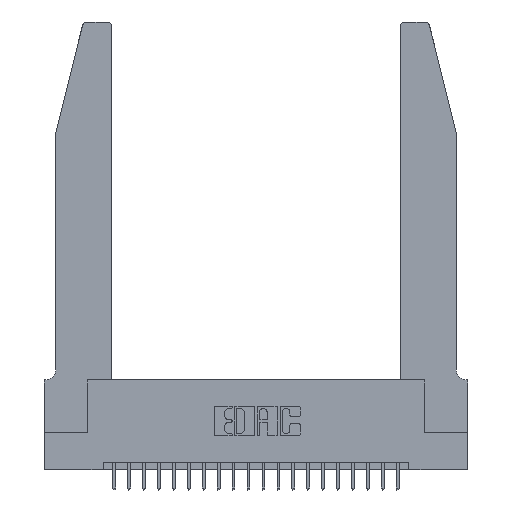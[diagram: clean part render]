
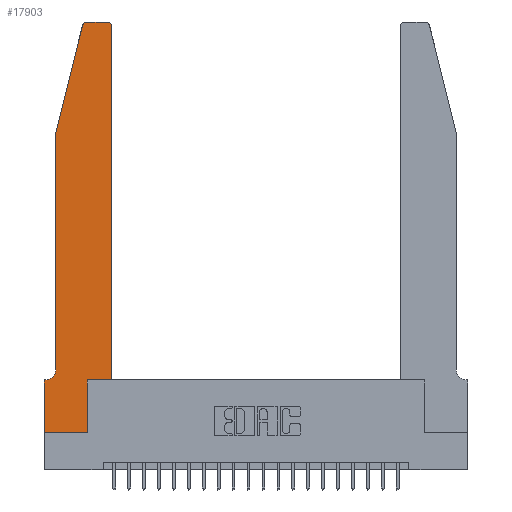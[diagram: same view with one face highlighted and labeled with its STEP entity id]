
A CAD part, top view. The second image highlights one B-rep face of the part: STEP entity #17903.
In plain terms, the highlighted planar face has unit normal (0, 0, 1).
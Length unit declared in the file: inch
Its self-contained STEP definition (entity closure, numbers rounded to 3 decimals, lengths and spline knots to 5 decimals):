
#9 = LINE ( 'NONE', #21988, #9299 ) ;
#37 = CARTESIAN_POINT ( 'NONE',  ( 0.284, 2.75, 0.37 ) ) ;
#168 = AXIS2_PLACEMENT_3D ( 'NONE', #8250, #23098, #8481 ) ;
#295 = AXIS2_PLACEMENT_3D ( 'NONE', #23239, #6489, #6945 ) ;
#527 = CARTESIAN_POINT ( 'NONE',  ( 0.4505, 0.35, 0.37 ) ) ;
#773 = DIRECTION ( 'NONE',  ( 0., -1., 0. ) ) ;
#843 = AXIS2_PLACEMENT_3D ( 'NONE', #21828, #7455, #3656 ) ;
#1049 = VERTEX_POINT ( 'NONE', #18879 ) ;
#1431 = LINE ( 'NONE', #8902, #14630 ) ;
#1601 = EDGE_CURVE ( 'NONE', #4205, #14137, #6245, .T. ) ;
#1781 = EDGE_CURVE ( 'NONE', #13615, #9035, #11203, .T. ) ;
#1956 = DIRECTION ( 'NONE',  ( 1., 0., 0. ) ) ;
#1986 = DIRECTION ( 'NONE',  ( 0., 1., 0. ) ) ;
#2216 = DIRECTION ( 'NONE',  ( 0., 1., 0. ) ) ;
#2668 = LINE ( 'NONE', #19183, #8946 ) ;
#3221 = EDGE_CURVE ( 'NONE', #9035, #3982, #1431, .T. ) ;
#3656 = DIRECTION ( 'NONE',  ( 1., 0., 0. ) ) ;
#3982 = VERTEX_POINT ( 'NONE', #9433 ) ;
#4205 = VERTEX_POINT ( 'NONE', #4580 ) ;
#4580 = CARTESIAN_POINT ( 'NONE',  ( 0.4505, 0.35, 0.37 ) ) ;
#4664 = EDGE_CURVE ( 'NONE', #1049, #4205, #9, .T. ) ;
#4724 = DIRECTION ( 'NONE',  ( 0., -1., 0. ) ) ;
#4725 = VERTEX_POINT ( 'NONE', #9026 ) ;
#5282 = ORIENTED_EDGE ( 'NONE', *, *, #1601, .T. ) ;
#6245 = LINE ( 'NONE', #527, #22203 ) ;
#6339 = VERTEX_POINT ( 'NONE', #8221 ) ;
#6489 = DIRECTION ( 'NONE',  ( 0., 0., 1. ) ) ;
#6945 = DIRECTION ( 'NONE',  ( 1., 0., 0. ) ) ;
#7062 = CARTESIAN_POINT ( 'NONE',  ( 0., 0.35, 0.37 ) ) ;
#7174 = LINE ( 'NONE', #11845, #17744 ) ;
#7227 = EDGE_CURVE ( 'NONE', #6339, #13615, #7174, .T. ) ;
#7356 = DIRECTION ( 'NONE',  ( 1., 0., 0. ) ) ;
#7357 = LINE ( 'NONE', #21075, #20033 ) ;
#7427 = CARTESIAN_POINT ( 'NONE',  ( 0.0755, 0.42, 0.37 ) ) ;
#7455 = DIRECTION ( 'NONE',  ( 0., 0., 1. ) ) ;
#7526 = AXIS2_PLACEMENT_3D ( 'NONE', #7062, #8830, #1956 ) ;
#7940 = EDGE_CURVE ( 'NONE', #14137, #8467, #21160, .T. ) ;
#8045 = CIRCLE ( 'NONE', #843, 0.03 ) ;
#8221 = CARTESIAN_POINT ( 'NONE',  ( 0.0755, 2., 0.37 ) ) ;
#8250 = CARTESIAN_POINT ( 'NONE',  ( 0.0055, 0.42, 0.37 ) ) ;
#8467 = VERTEX_POINT ( 'NONE', #19097 ) ;
#8481 = DIRECTION ( 'NONE',  ( -1., 0., 0. ) ) ;
#8628 = LINE ( 'NONE', #17665, #11826 ) ;
#8756 = ORIENTED_EDGE ( 'NONE', *, *, #1781, .T. ) ;
#8830 = DIRECTION ( 'NONE',  ( 0., 0., 1. ) ) ;
#8902 = CARTESIAN_POINT ( 'NONE',  ( 0.0755, 0.35, 0.37 ) ) ;
#8946 = VECTOR ( 'NONE', #773, 39.37008 ) ;
#9026 = CARTESIAN_POINT ( 'NONE',  ( 0., 0., 0.37 ) ) ;
#9035 = VERTEX_POINT ( 'NONE', #15468 ) ;
#9197 = EDGE_CURVE ( 'NONE', #4725, #21643, #20291, .T. ) ;
#9299 = VECTOR ( 'NONE', #14511, 39.37008 ) ;
#9433 = CARTESIAN_POINT ( 'NONE',  ( 0., 0.35, 0.37 ) ) ;
#9518 = VECTOR ( 'NONE', #20572, 39.37008 ) ;
#10030 = EDGE_LOOP ( 'NONE', ( #13180, #12534, #22954, #17304, #8756, #23449, #12847, #22909, #19371, #20914, #5282, #10141 ) ) ;
#10141 = ORIENTED_EDGE ( 'NONE', *, *, #7940, .T. ) ;
#10971 = VECTOR ( 'NONE', #7356, 39.37008 ) ;
#11203 = CIRCLE ( 'NONE', #168, 0.07 ) ;
#11826 = VECTOR ( 'NONE', #1986, 39.37008 ) ;
#11845 = CARTESIAN_POINT ( 'NONE',  ( 0.0755, 2., 0.37 ) ) ;
#12018 = DIRECTION ( 'NONE',  ( -1., 0., 0. ) ) ;
#12534 = ORIENTED_EDGE ( 'NONE', *, *, #14571, .T. ) ;
#12847 = ORIENTED_EDGE ( 'NONE', *, *, #15275, .T. ) ;
#13180 = ORIENTED_EDGE ( 'NONE', *, *, #23106, .T. ) ;
#13610 = DIRECTION ( 'NONE',  ( -0.239, -0.971, 0. ) ) ;
#13615 = VERTEX_POINT ( 'NONE', #7427 ) ;
#13830 = EDGE_CURVE ( 'NONE', #21643, #1049, #8628, .T. ) ;
#13940 = CARTESIAN_POINT ( 'NONE',  ( 0.2865, 0., 0.37 ) ) ;
#14137 = VERTEX_POINT ( 'NONE', #20413 ) ;
#14424 = FACE_OUTER_BOUND ( 'NONE', #10030, .T. ) ;
#14511 = DIRECTION ( 'NONE',  ( 1., 0., 0. ) ) ;
#14571 = EDGE_CURVE ( 'NONE', #15580, #19890, #8045, .T. ) ;
#14630 = VECTOR ( 'NONE', #12018, 39.37008 ) ;
#15275 = EDGE_CURVE ( 'NONE', #3982, #4725, #2668, .T. ) ;
#15468 = CARTESIAN_POINT ( 'NONE',  ( 0.0055, 0.35, 0.37 ) ) ;
#15580 = VERTEX_POINT ( 'NONE', #37 ) ;
#17008 = LINE ( 'NONE', #22490, #9518 ) ;
#17304 = ORIENTED_EDGE ( 'NONE', *, *, #7227, .T. ) ;
#17665 = CARTESIAN_POINT ( 'NONE',  ( 0.2865, 0.35, 0.37 ) ) ;
#17728 = EDGE_CURVE ( 'NONE', #19890, #6339, #7357, .T. ) ;
#17744 = VECTOR ( 'NONE', #4724, 39.37008 ) ;
#17903 = ADVANCED_FACE ( 'NONE', ( #14424 ), #18104, .T. ) ;
#18104 = PLANE ( 'NONE',  #7526 ) ;
#18160 = CARTESIAN_POINT ( 'NONE',  ( 0., 0., 0.37 ) ) ;
#18879 = CARTESIAN_POINT ( 'NONE',  ( 0.2865, 0.35, 0.37 ) ) ;
#19097 = CARTESIAN_POINT ( 'NONE',  ( 0.4205, 2.75, 0.37 ) ) ;
#19183 = CARTESIAN_POINT ( 'NONE',  ( 0., 0., 0.37 ) ) ;
#19371 = ORIENTED_EDGE ( 'NONE', *, *, #13830, .T. ) ;
#19890 = VERTEX_POINT ( 'NONE', #21194 ) ;
#20033 = VECTOR ( 'NONE', #13610, 39.37008 ) ;
#20291 = LINE ( 'NONE', #18160, #10971 ) ;
#20413 = CARTESIAN_POINT ( 'NONE',  ( 0.4505, 2.72, 0.37 ) ) ;
#20572 = DIRECTION ( 'NONE',  ( -1., 0., 0. ) ) ;
#20914 = ORIENTED_EDGE ( 'NONE', *, *, #4664, .T. ) ;
#21075 = CARTESIAN_POINT ( 'NONE',  ( 0.0755, 2., 0.37 ) ) ;
#21160 = CIRCLE ( 'NONE', #295, 0.03 ) ;
#21194 = CARTESIAN_POINT ( 'NONE',  ( 0.25487, 2.72718, 0.37 ) ) ;
#21643 = VERTEX_POINT ( 'NONE', #13940 ) ;
#21828 = CARTESIAN_POINT ( 'NONE',  ( 0.284, 2.72, 0.37 ) ) ;
#21988 = CARTESIAN_POINT ( 'NONE',  ( 0.4505, 0.35, 0.37 ) ) ;
#22203 = VECTOR ( 'NONE', #2216, 39.37008 ) ;
#22490 = CARTESIAN_POINT ( 'NONE',  ( 0.2605, 2.75, 0.37 ) ) ;
#22909 = ORIENTED_EDGE ( 'NONE', *, *, #9197, .T. ) ;
#22954 = ORIENTED_EDGE ( 'NONE', *, *, #17728, .T. ) ;
#23098 = DIRECTION ( 'NONE',  ( 0., 0., -1. ) ) ;
#23106 = EDGE_CURVE ( 'NONE', #8467, #15580, #17008, .T. ) ;
#23239 = CARTESIAN_POINT ( 'NONE',  ( 0.4205, 2.72, 0.37 ) ) ;
#23449 = ORIENTED_EDGE ( 'NONE', *, *, #3221, .T. ) ;
